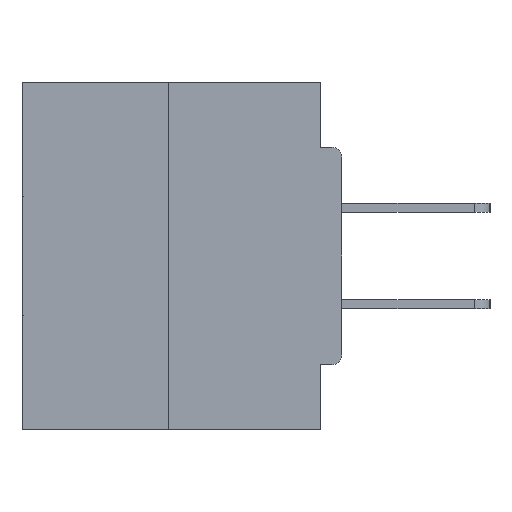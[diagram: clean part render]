
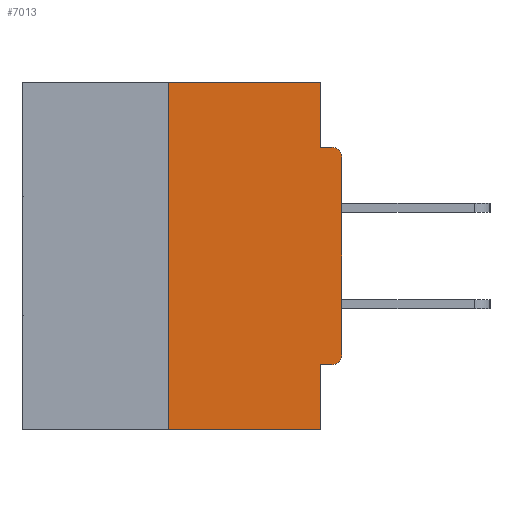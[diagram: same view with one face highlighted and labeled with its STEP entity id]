
A CAD part, left-side view. The second image highlights one B-rep face of the part: STEP entity #7013.
In plain terms, the highlighted planar face has unit normal (-1, 0, 0).
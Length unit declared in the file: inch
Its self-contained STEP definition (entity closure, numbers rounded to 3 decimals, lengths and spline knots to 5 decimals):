
#658 = CIRCLE ( 'NONE', #6196, 0.015 ) ;
#763 = DIRECTION ( 'NONE',  ( 0., 0., -1. ) ) ;
#1090 = CARTESIAN_POINT ( 'NONE',  ( 0., 0., 0. ) ) ;
#1175 = VERTEX_POINT ( 'NONE', #2921 ) ;
#2724 = VERTEX_POINT ( 'NONE', #7758 ) ;
#2732 = LINE ( 'NONE', #4756, #4104 ) ;
#2900 = EDGE_CURVE ( 'NONE', #19812, #4374, #658, .T. ) ;
#2921 = CARTESIAN_POINT ( 'NONE',  ( 0., 0.25, -0.5 ) ) ;
#3109 = DIRECTION ( 'NONE',  ( 0., 0., -1. ) ) ;
#3503 = DIRECTION ( 'NONE',  ( -1., 0., 0. ) ) ;
#3515 = ORIENTED_EDGE ( 'NONE', *, *, #21500, .F. ) ;
#3604 = FACE_OUTER_BOUND ( 'NONE', #31281, .T. ) ;
#3801 = CARTESIAN_POINT ( 'NONE',  ( 0., 0.46, -0.5 ) ) ;
#4104 = VECTOR ( 'NONE', #4364, 39.37008 ) ;
#4364 = DIRECTION ( 'NONE',  ( 0., 0., -1. ) ) ;
#4374 = VERTEX_POINT ( 'NONE', #13611 ) ;
#4752 = DIRECTION ( 'NONE',  ( 0., 0., -1. ) ) ;
#4756 = CARTESIAN_POINT ( 'NONE',  ( 0., 0.031, -0.5 ) ) ;
#5302 = DIRECTION ( 'NONE',  ( 0., -1., 0. ) ) ;
#5408 = VERTEX_POINT ( 'NONE', #17375 ) ;
#5596 = CARTESIAN_POINT ( 'NONE',  ( 0., 0.25, 0. ) ) ;
#5634 = VECTOR ( 'NONE', #32340, 39.37008 ) ;
#6196 = AXIS2_PLACEMENT_3D ( 'NONE', #26572, #3503, #3109 ) ;
#6375 = CARTESIAN_POINT ( 'NONE',  ( 0., 0.015, -0.3915 ) ) ;
#7013 = ADVANCED_FACE ( 'NONE', ( #3604 ), #14275, .F. ) ;
#7264 = VECTOR ( 'NONE', #14979, 39.37008 ) ;
#7758 = CARTESIAN_POINT ( 'NONE',  ( 0., 0., -0.3915 ) ) ;
#7971 = VECTOR ( 'NONE', #24528, 39.37008 ) ;
#8529 = LINE ( 'NONE', #23241, #13143 ) ;
#8661 = AXIS2_PLACEMENT_3D ( 'NONE', #6375, #35288, #35426 ) ;
#10518 = ORIENTED_EDGE ( 'NONE', *, *, #2900, .T. ) ;
#11171 = VECTOR ( 'NONE', #5302, 39.37008 ) ;
#12176 = VECTOR ( 'NONE', #22348, 39.37008 ) ;
#12747 = EDGE_CURVE ( 'NONE', #29328, #4374, #36899, .T. ) ;
#13143 = VECTOR ( 'NONE', #26108, 39.37008 ) ;
#13611 = CARTESIAN_POINT ( 'NONE',  ( 0., 0.015, -0.0935 ) ) ;
#13680 = EDGE_CURVE ( 'NONE', #25942, #2724, #25956, .T. ) ;
#14275 = PLANE ( 'NONE',  #34372 ) ;
#14527 = CARTESIAN_POINT ( 'NONE',  ( 0., 0.46, 0. ) ) ;
#14720 = VERTEX_POINT ( 'NONE', #28239 ) ;
#14979 = DIRECTION ( 'NONE',  ( 0., -1., 0. ) ) ;
#16142 = ORIENTED_EDGE ( 'NONE', *, *, #27744, .F. ) ;
#16864 = CARTESIAN_POINT ( 'NONE',  ( 0., 0.46, 0. ) ) ;
#17375 = CARTESIAN_POINT ( 'NONE',  ( 0., 0.031, -0.5 ) ) ;
#17789 = LINE ( 'NONE', #34405, #28308 ) ;
#18040 = LINE ( 'NONE', #1090, #7971 ) ;
#18737 = CARTESIAN_POINT ( 'NONE',  ( 0., 0.031, 0. ) ) ;
#19195 = EDGE_CURVE ( 'NONE', #1175, #5408, #20535, .T. ) ;
#19738 = VERTEX_POINT ( 'NONE', #18737 ) ;
#19812 = VERTEX_POINT ( 'NONE', #33629 ) ;
#20523 = ORIENTED_EDGE ( 'NONE', *, *, #35705, .T. ) ;
#20535 = LINE ( 'NONE', #3801, #7264 ) ;
#20796 = DIRECTION ( 'NONE',  ( 1., 0., 0. ) ) ;
#21500 = EDGE_CURVE ( 'NONE', #25942, #36712, #8529, .T. ) ;
#21786 = LINE ( 'NONE', #5596, #12176 ) ;
#22348 = DIRECTION ( 'NONE',  ( 0., 0., 1. ) ) ;
#22509 = EDGE_CURVE ( 'NONE', #14720, #19738, #30905, .T. ) ;
#23241 = CARTESIAN_POINT ( 'NONE',  ( 0., 0., -0.4065 ) ) ;
#24528 = DIRECTION ( 'NONE',  ( 0., 0., 1. ) ) ;
#25192 = EDGE_CURVE ( 'NONE', #36712, #5408, #2732, .T. ) ;
#25194 = ORIENTED_EDGE ( 'NONE', *, *, #31937, .F. ) ;
#25450 = ORIENTED_EDGE ( 'NONE', *, *, #22509, .F. ) ;
#25942 = VERTEX_POINT ( 'NONE', #32466 ) ;
#25956 = CIRCLE ( 'NONE', #8661, 0.015 ) ;
#26108 = DIRECTION ( 'NONE',  ( 0., 1., 0. ) ) ;
#26572 = CARTESIAN_POINT ( 'NONE',  ( 0., 0.015, -0.1085 ) ) ;
#27744 = EDGE_CURVE ( 'NONE', #1175, #14720, #21786, .T. ) ;
#28239 = CARTESIAN_POINT ( 'NONE',  ( 0., 0.25, 0. ) ) ;
#28308 = VECTOR ( 'NONE', #4752, 39.37008 ) ;
#29328 = VERTEX_POINT ( 'NONE', #33621 ) ;
#29887 = CARTESIAN_POINT ( 'NONE',  ( 0., 0., -0.0935 ) ) ;
#30313 = ORIENTED_EDGE ( 'NONE', *, *, #25192, .F. ) ;
#30633 = ORIENTED_EDGE ( 'NONE', *, *, #19195, .T. ) ;
#30905 = LINE ( 'NONE', #16864, #11171 ) ;
#31281 = EDGE_LOOP ( 'NONE', ( #25450, #16142, #30633, #30313, #3515, #34054, #20523, #10518, #34999, #25194 ) ) ;
#31937 = EDGE_CURVE ( 'NONE', #19738, #29328, #17789, .T. ) ;
#32340 = DIRECTION ( 'NONE',  ( 0., -1., 0. ) ) ;
#32466 = CARTESIAN_POINT ( 'NONE',  ( 0., 0.015, -0.4065 ) ) ;
#33621 = CARTESIAN_POINT ( 'NONE',  ( 0., 0.031, -0.0935 ) ) ;
#33629 = CARTESIAN_POINT ( 'NONE',  ( 0., 0., -0.1085 ) ) ;
#34054 = ORIENTED_EDGE ( 'NONE', *, *, #13680, .T. ) ;
#34372 = AXIS2_PLACEMENT_3D ( 'NONE', #14527, #20796, #763 ) ;
#34405 = CARTESIAN_POINT ( 'NONE',  ( 0., 0.031, 0. ) ) ;
#34999 = ORIENTED_EDGE ( 'NONE', *, *, #12747, .F. ) ;
#35288 = DIRECTION ( 'NONE',  ( -1., 0., 0. ) ) ;
#35426 = DIRECTION ( 'NONE',  ( 0., 0., -1. ) ) ;
#35432 = CARTESIAN_POINT ( 'NONE',  ( 0., 0.031, -0.4065 ) ) ;
#35705 = EDGE_CURVE ( 'NONE', #2724, #19812, #18040, .T. ) ;
#36712 = VERTEX_POINT ( 'NONE', #35432 ) ;
#36899 = LINE ( 'NONE', #29887, #5634 ) ;
